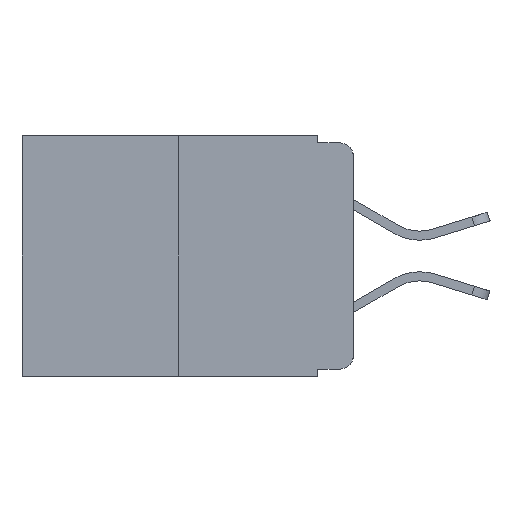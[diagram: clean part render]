
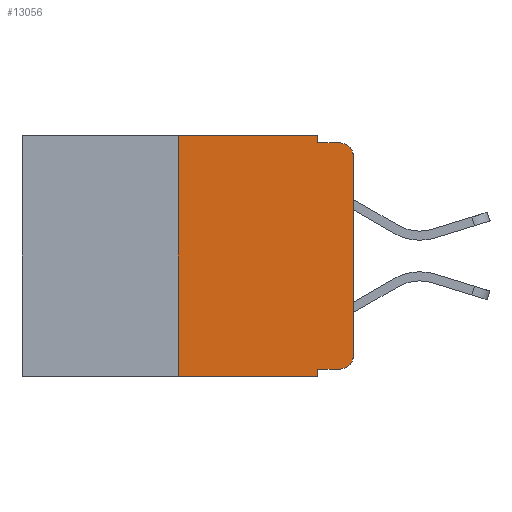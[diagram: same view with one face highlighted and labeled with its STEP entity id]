
A CAD part, left-side view. The second image highlights one B-rep face of the part: STEP entity #13056.
In plain terms, the highlighted planar face has unit normal (-1, 0, 0).
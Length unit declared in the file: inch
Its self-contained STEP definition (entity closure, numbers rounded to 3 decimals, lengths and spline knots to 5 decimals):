
#499 = CARTESIAN_POINT ( 'NONE',  ( 0., 0.473, 0. ) ) ;
#548 = CARTESIAN_POINT ( 'NONE',  ( 0., 0.051, -0.01 ) ) ;
#772 = VERTEX_POINT ( 'NONE', #11398 ) ;
#910 = VERTEX_POINT ( 'NONE', #8711 ) ;
#1020 = EDGE_CURVE ( 'NONE', #910, #3788, #2583, .T. ) ;
#1046 = DIRECTION ( 'NONE',  ( 0., 0., -1. ) ) ;
#1183 = LINE ( 'NONE', #15780, #10859 ) ;
#1837 = DIRECTION ( 'NONE',  ( 0., -1., 0. ) ) ;
#2247 = DIRECTION ( 'NONE',  ( 0., -1., 0. ) ) ;
#2298 = VERTEX_POINT ( 'NONE', #7301 ) ;
#2583 = LINE ( 'NONE', #548, #8902 ) ;
#3203 = FACE_OUTER_BOUND ( 'NONE', #3604, .T. ) ;
#3292 = VERTEX_POINT ( 'NONE', #7876 ) ;
#3398 = DIRECTION ( 'NONE',  ( 1., 0., 0. ) ) ;
#3604 = EDGE_LOOP ( 'NONE', ( #12867, #15103, #11837, #16021, #14125, #10824, #4693, #14164, #13601, #12118 ) ) ;
#3788 = VERTEX_POINT ( 'NONE', #11491 ) ;
#3795 = CARTESIAN_POINT ( 'NONE',  ( 0., 0.02, -0.333 ) ) ;
#4025 = EDGE_CURVE ( 'NONE', #14451, #5946, #12552, .T. ) ;
#4143 = CIRCLE ( 'NONE', #11467, 0.02 ) ;
#4510 = VERTEX_POINT ( 'NONE', #15630 ) ;
#4693 = ORIENTED_EDGE ( 'NONE', *, *, #5285, .T. ) ;
#5016 = VECTOR ( 'NONE', #7184, 39.37008 ) ;
#5285 = EDGE_CURVE ( 'NONE', #772, #3292, #12198, .T. ) ;
#5388 = EDGE_CURVE ( 'NONE', #6269, #3788, #4143, .T. ) ;
#5946 = VERTEX_POINT ( 'NONE', #9880 ) ;
#6269 = VERTEX_POINT ( 'NONE', #11732 ) ;
#6303 = AXIS2_PLACEMENT_3D ( 'NONE', #13909, #6729, #15092 ) ;
#6557 = DIRECTION ( 'NONE',  ( -1., 0., 0. ) ) ;
#6729 = DIRECTION ( 'NONE',  ( -1., 0., 0. ) ) ;
#7068 = EDGE_CURVE ( 'NONE', #4510, #6269, #11557, .T. ) ;
#7156 = CARTESIAN_POINT ( 'NONE',  ( 0., 0.051, 0. ) ) ;
#7184 = DIRECTION ( 'NONE',  ( 0., 0., 1. ) ) ;
#7301 = CARTESIAN_POINT ( 'NONE',  ( 0., 0.051, -0.333 ) ) ;
#7513 = CIRCLE ( 'NONE', #6303, 0.02 ) ;
#7876 = CARTESIAN_POINT ( 'NONE',  ( 0., 0.051, -0.343 ) ) ;
#7973 = EDGE_CURVE ( 'NONE', #9514, #4510, #7513, .T. ) ;
#8368 = VECTOR ( 'NONE', #8376, 39.37008 ) ;
#8376 = DIRECTION ( 'NONE',  ( 0., 0., -1. ) ) ;
#8388 = PLANE ( 'NONE',  #12233 ) ;
#8711 = CARTESIAN_POINT ( 'NONE',  ( 0., 0.051, -0.01 ) ) ;
#8836 = CARTESIAN_POINT ( 'NONE',  ( 0., 0.25, 0. ) ) ;
#8902 = VECTOR ( 'NONE', #2247, 39.37008 ) ;
#9000 = LINE ( 'NONE', #13760, #12550 ) ;
#9109 = CARTESIAN_POINT ( 'NONE',  ( 0., 0.25, 0. ) ) ;
#9387 = VECTOR ( 'NONE', #1837, 39.37008 ) ;
#9514 = VERTEX_POINT ( 'NONE', #3795 ) ;
#9613 = EDGE_CURVE ( 'NONE', #2298, #9514, #9000, .T. ) ;
#9880 = CARTESIAN_POINT ( 'NONE',  ( 0., 0.051, 0. ) ) ;
#10687 = LINE ( 'NONE', #9109, #13046 ) ;
#10824 = ORIENTED_EDGE ( 'NONE', *, *, #14588, .F. ) ;
#10859 = VECTOR ( 'NONE', #1046, 39.37008 ) ;
#10864 = CARTESIAN_POINT ( 'NONE',  ( 0., 0.473, 0. ) ) ;
#11221 = CARTESIAN_POINT ( 'NONE',  ( 0., 0.473, -0.343 ) ) ;
#11252 = EDGE_CURVE ( 'NONE', #2298, #3292, #1183, .T. ) ;
#11398 = CARTESIAN_POINT ( 'NONE',  ( 0., 0.25, -0.343 ) ) ;
#11441 = DIRECTION ( 'NONE',  ( 0., -1., 0. ) ) ;
#11467 = AXIS2_PLACEMENT_3D ( 'NONE', #13741, #6557, #14927 ) ;
#11491 = CARTESIAN_POINT ( 'NONE',  ( 0., 0.02, -0.01 ) ) ;
#11551 = DIRECTION ( 'NONE',  ( 0., 0., 1. ) ) ;
#11557 = LINE ( 'NONE', #15540, #5016 ) ;
#11614 = LINE ( 'NONE', #7156, #8368 ) ;
#11732 = CARTESIAN_POINT ( 'NONE',  ( 0., 0., -0.03 ) ) ;
#11834 = VECTOR ( 'NONE', #15859, 39.37008 ) ;
#11837 = ORIENTED_EDGE ( 'NONE', *, *, #1020, .F. ) ;
#12045 = DIRECTION ( 'NONE',  ( 0., 0., -1. ) ) ;
#12118 = ORIENTED_EDGE ( 'NONE', *, *, #7973, .T. ) ;
#12198 = LINE ( 'NONE', #11221, #11834 ) ;
#12233 = AXIS2_PLACEMENT_3D ( 'NONE', #10864, #3398, #12045 ) ;
#12550 = VECTOR ( 'NONE', #11441, 39.37008 ) ;
#12552 = LINE ( 'NONE', #499, #9387 ) ;
#12867 = ORIENTED_EDGE ( 'NONE', *, *, #7068, .T. ) ;
#13046 = VECTOR ( 'NONE', #11551, 39.37008 ) ;
#13056 = ADVANCED_FACE ( 'NONE', ( #3203 ), #8388, .F. ) ;
#13601 = ORIENTED_EDGE ( 'NONE', *, *, #9613, .T. ) ;
#13741 = CARTESIAN_POINT ( 'NONE',  ( 0., 0.02, -0.03 ) ) ;
#13760 = CARTESIAN_POINT ( 'NONE',  ( 0., 0.051, -0.333 ) ) ;
#13909 = CARTESIAN_POINT ( 'NONE',  ( 0., 0.02, -0.313 ) ) ;
#14125 = ORIENTED_EDGE ( 'NONE', *, *, #4025, .F. ) ;
#14164 = ORIENTED_EDGE ( 'NONE', *, *, #11252, .F. ) ;
#14451 = VERTEX_POINT ( 'NONE', #8836 ) ;
#14588 = EDGE_CURVE ( 'NONE', #772, #14451, #10687, .T. ) ;
#14927 = DIRECTION ( 'NONE',  ( 0., 0., -1. ) ) ;
#15092 = DIRECTION ( 'NONE',  ( 0., 0., -1. ) ) ;
#15103 = ORIENTED_EDGE ( 'NONE', *, *, #5388, .T. ) ;
#15385 = EDGE_CURVE ( 'NONE', #5946, #910, #11614, .T. ) ;
#15540 = CARTESIAN_POINT ( 'NONE',  ( 0., 0., 0. ) ) ;
#15630 = CARTESIAN_POINT ( 'NONE',  ( 0., 0., -0.313 ) ) ;
#15780 = CARTESIAN_POINT ( 'NONE',  ( 0., 0.051, 0. ) ) ;
#15859 = DIRECTION ( 'NONE',  ( 0., -1., 0. ) ) ;
#16021 = ORIENTED_EDGE ( 'NONE', *, *, #15385, .F. ) ;
